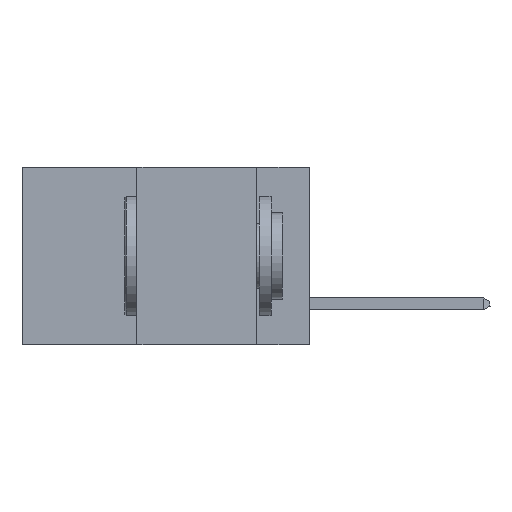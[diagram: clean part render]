
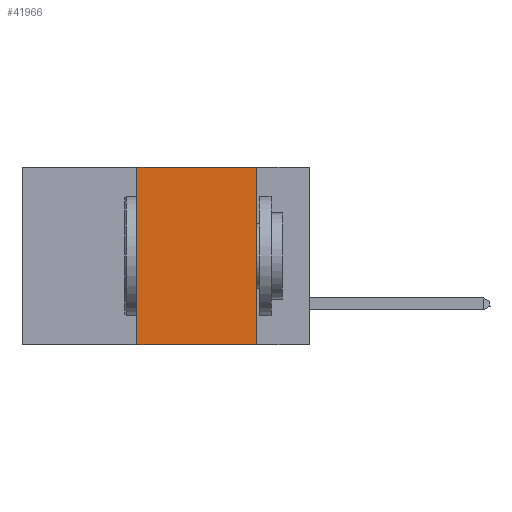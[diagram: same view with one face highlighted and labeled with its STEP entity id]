
A CAD part, left-side view. The second image highlights one B-rep face of the part: STEP entity #41966.
In plain terms, the highlighted planar face has unit normal (-1, 0, 0).
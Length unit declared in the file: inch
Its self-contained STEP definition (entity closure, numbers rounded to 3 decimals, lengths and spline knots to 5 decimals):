
#847 = CARTESIAN_POINT ( 'NONE',  ( 0., 0.11, 0. ) ) ;
#999 = VERTEX_POINT ( 'NONE', #21911 ) ;
#2174 = VECTOR ( 'NONE', #8360, 39.37008 ) ;
#3892 = VECTOR ( 'NONE', #10552, 39.37008 ) ;
#4365 = ORIENTED_EDGE ( 'NONE', *, *, #48877, .F. ) ;
#5474 = PLANE ( 'NONE',  #5959 ) ;
#5959 = AXIS2_PLACEMENT_3D ( 'NONE', #47590, #9293, #36320 ) ;
#8151 = LINE ( 'NONE', #24263, #45460 ) ;
#8360 = DIRECTION ( 'NONE',  ( 0., 0., -1. ) ) ;
#9293 = DIRECTION ( 'NONE',  ( 1., 0., 0. ) ) ;
#10552 = DIRECTION ( 'NONE',  ( 0., -1., 0. ) ) ;
#10835 = VERTEX_POINT ( 'NONE', #37693 ) ;
#12459 = ORIENTED_EDGE ( 'NONE', *, *, #19532, .F. ) ;
#15908 = VERTEX_POINT ( 'NONE', #24604 ) ;
#16220 = ORIENTED_EDGE ( 'NONE', *, *, #38964, .T. ) ;
#16944 = VECTOR ( 'NONE', #16957, 39.37008 ) ;
#16957 = DIRECTION ( 'NONE',  ( 0., 0., 1. ) ) ;
#17363 = VERTEX_POINT ( 'NONE', #19308 ) ;
#17775 = LINE ( 'NONE', #48792, #3892 ) ;
#19308 = CARTESIAN_POINT ( 'NONE',  ( 0., 0.36, 0. ) ) ;
#19532 = EDGE_CURVE ( 'NONE', #10835, #17363, #38606, .T. ) ;
#21911 = CARTESIAN_POINT ( 'NONE',  ( 0., 0.11, -0.37 ) ) ;
#24263 = CARTESIAN_POINT ( 'NONE',  ( 0., 0.6, 0. ) ) ;
#24604 = CARTESIAN_POINT ( 'NONE',  ( 0., 0.11, 0. ) ) ;
#25377 = ORIENTED_EDGE ( 'NONE', *, *, #35773, .F. ) ;
#29071 = FACE_OUTER_BOUND ( 'NONE', #41084, .T. ) ;
#31756 = LINE ( 'NONE', #847, #2174 ) ;
#34488 = DIRECTION ( 'NONE',  ( 0., -1., 0. ) ) ;
#35773 = EDGE_CURVE ( 'NONE', #15908, #999, #31756, .T. ) ;
#36320 = DIRECTION ( 'NONE',  ( 0., 0., -1. ) ) ;
#37693 = CARTESIAN_POINT ( 'NONE',  ( 0., 0.36, -0.37 ) ) ;
#38606 = LINE ( 'NONE', #39997, #16944 ) ;
#38964 = EDGE_CURVE ( 'NONE', #10835, #999, #17775, .T. ) ;
#39997 = CARTESIAN_POINT ( 'NONE',  ( 0., 0.36, 0. ) ) ;
#41084 = EDGE_LOOP ( 'NONE', ( #25377, #4365, #12459, #16220 ) ) ;
#41966 = ADVANCED_FACE ( 'NONE', ( #29071 ), #5474, .F. ) ;
#45460 = VECTOR ( 'NONE', #34488, 39.37008 ) ;
#47590 = CARTESIAN_POINT ( 'NONE',  ( 0., 0.6, 0. ) ) ;
#48792 = CARTESIAN_POINT ( 'NONE',  ( 0., 0.6, -0.37 ) ) ;
#48877 = EDGE_CURVE ( 'NONE', #17363, #15908, #8151, .T. ) ;
